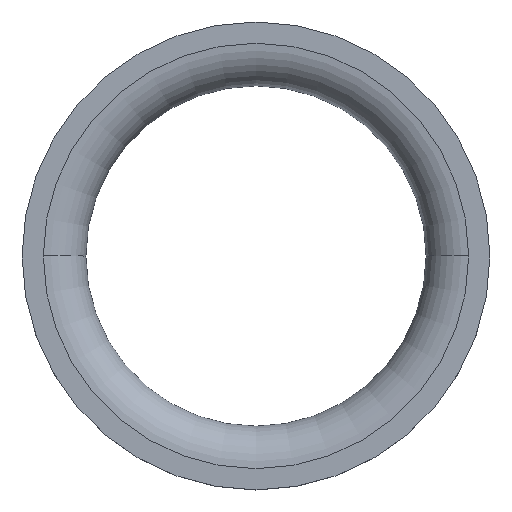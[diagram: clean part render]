
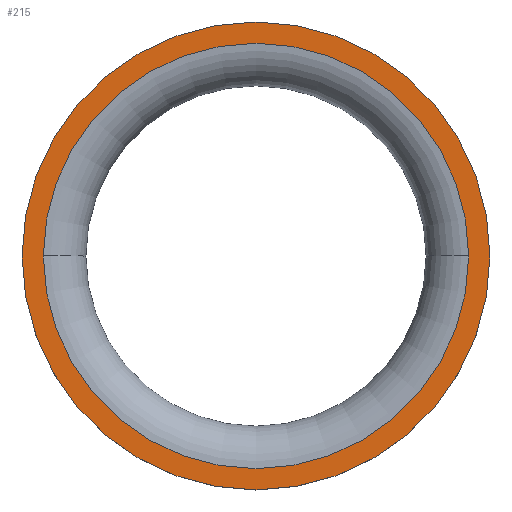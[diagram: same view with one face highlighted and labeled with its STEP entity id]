
A CAD part, top view. The second image highlights one B-rep face of the part: STEP entity #215.
In plain terms, the highlighted planar face has unit normal (0, 0, 1).
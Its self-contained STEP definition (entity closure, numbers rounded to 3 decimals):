
#14 = DIRECTION ( 'NONE',  ( 0., 0., 1. ) ) ;
#26 = FACE_OUTER_BOUND ( 'NONE', #76, .T. ) ;
#32 = FACE_BOUND ( 'NONE', #149, .T. ) ;
#47 = ORIENTED_EDGE ( 'NONE', *, *, #238, .T. ) ;
#48 = ORIENTED_EDGE ( 'NONE', *, *, #259, .T. ) ;
#52 = CARTESIAN_POINT ( 'NONE',  ( 0., 0., 1.27 ) ) ;
#53 = ORIENTED_EDGE ( 'NONE', *, *, #232, .T. ) ;
#61 = CARTESIAN_POINT ( 'NONE',  ( -5.588, 0., 1.27 ) ) ;
#63 = PLANE ( 'NONE',  #206 ) ;
#67 = DIRECTION ( 'NONE',  ( 0., 0., -1. ) ) ;
#75 = ORIENTED_EDGE ( 'NONE', *, *, #250, .T. ) ;
#76 = EDGE_LOOP ( 'NONE', ( #75, #47 ) ) ;
#77 = DIRECTION ( 'NONE',  ( 0., 0., 1. ) ) ;
#81 = CARTESIAN_POINT ( 'NONE',  ( -5.08, 0., 1.27 ) ) ;
#93 = CIRCLE ( 'NONE', #178, 5.08 ) ;
#104 = VERTEX_POINT ( 'NONE', #182 ) ;
#105 = DIRECTION ( 'NONE',  ( 1., 0., 0. ) ) ;
#121 = CARTESIAN_POINT ( 'NONE',  ( 0., 0., 1.27 ) ) ;
#130 = VERTEX_POINT ( 'NONE', #61 ) ;
#139 = VERTEX_POINT ( 'NONE', #233 ) ;
#149 = EDGE_LOOP ( 'NONE', ( #53, #48 ) ) ;
#155 = VERTEX_POINT ( 'NONE', #81 ) ;
#166 = CIRCLE ( 'NONE', #201, 5.08 ) ;
#178 = AXIS2_PLACEMENT_3D ( 'NONE', #255, #251, #246 ) ;
#182 = CARTESIAN_POINT ( 'NONE',  ( 5.588, 0., 1.27 ) ) ;
#185 = AXIS2_PLACEMENT_3D ( 'NONE', #224, #222, #194 ) ;
#189 = DIRECTION ( 'NONE',  ( 1., 0., 0. ) ) ;
#193 = DIRECTION ( 'NONE',  ( 1., 0., 0. ) ) ;
#194 = DIRECTION ( 'NONE',  ( 1., 0., 0. ) ) ;
#195 = AXIS2_PLACEMENT_3D ( 'NONE', #121, #14, #105 ) ;
#201 = AXIS2_PLACEMENT_3D ( 'NONE', #240, #67, #193 ) ;
#206 = AXIS2_PLACEMENT_3D ( 'NONE', #52, #77, #189 ) ;
#215 = ADVANCED_FACE ( 'NONE', ( #32, #26 ), #63, .T. ) ;
#222 = DIRECTION ( 'NONE',  ( 0., 0., 1. ) ) ;
#224 = CARTESIAN_POINT ( 'NONE',  ( 0., 0., 1.27 ) ) ;
#232 = EDGE_CURVE ( 'NONE', #139, #155, #166, .T. ) ;
#233 = CARTESIAN_POINT ( 'NONE',  ( 5.08, 0., 1.27 ) ) ;
#238 = EDGE_CURVE ( 'NONE', #104, #130, #241, .T. ) ;
#240 = CARTESIAN_POINT ( 'NONE',  ( 0., 0., 1.27 ) ) ;
#241 = CIRCLE ( 'NONE', #195, 5.588 ) ;
#246 = DIRECTION ( 'NONE',  ( 1., 0., 0. ) ) ;
#250 = EDGE_CURVE ( 'NONE', #130, #104, #257, .T. ) ;
#251 = DIRECTION ( 'NONE',  ( 0., 0., -1. ) ) ;
#255 = CARTESIAN_POINT ( 'NONE',  ( 0., 0., 1.27 ) ) ;
#257 = CIRCLE ( 'NONE', #185, 5.588 ) ;
#259 = EDGE_CURVE ( 'NONE', #155, #139, #93, .T. ) ;
